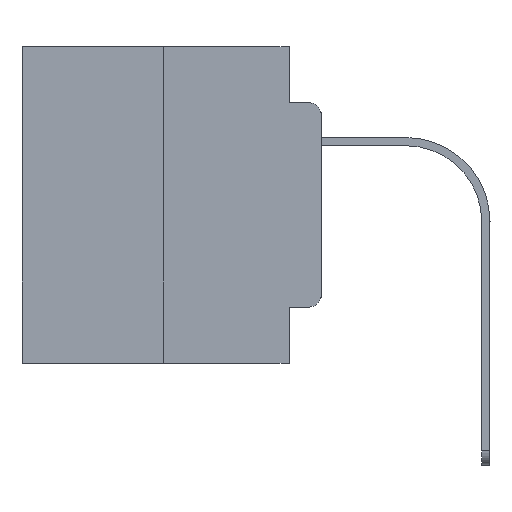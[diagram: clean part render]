
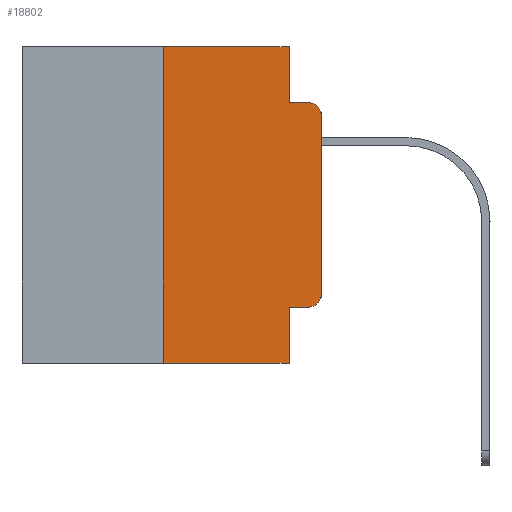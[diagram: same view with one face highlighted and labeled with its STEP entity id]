
A CAD part, left-side view. The second image highlights one B-rep face of the part: STEP entity #18802.
In plain terms, the highlighted planar face has unit normal (-1, 0, 0).
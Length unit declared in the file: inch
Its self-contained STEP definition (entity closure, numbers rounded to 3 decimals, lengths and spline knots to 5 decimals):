
#91 = AXIS2_PLACEMENT_3D ( 'NONE', #1571, #3238, #13882 ) ;
#158 = LINE ( 'NONE', #8084, #26917 ) ;
#404 = EDGE_CURVE ( 'NONE', #3718, #3940, #21538, .T. ) ;
#651 = CARTESIAN_POINT ( 'NONE',  ( 0., 0.051, -0.0885 ) ) ;
#1571 = CARTESIAN_POINT ( 'NONE',  ( 0., 0.02, -0.1085 ) ) ;
#2907 = CARTESIAN_POINT ( 'NONE',  ( 0., 0.051, 0. ) ) ;
#2915 = VECTOR ( 'NONE', #13723, 39.37008 ) ;
#3058 = DIRECTION ( 'NONE',  ( 0., 0., -1. ) ) ;
#3238 = DIRECTION ( 'NONE',  ( -1., 0., 0. ) ) ;
#3377 = LINE ( 'NONE', #20069, #20087 ) ;
#3543 = VECTOR ( 'NONE', #8685, 39.37008 ) ;
#3655 = DIRECTION ( 'NONE',  ( 0., 0., 1. ) ) ;
#3718 = VERTEX_POINT ( 'NONE', #19006 ) ;
#3940 = VERTEX_POINT ( 'NONE', #14063 ) ;
#4103 = EDGE_LOOP ( 'NONE', ( #11067, #22926, #19680, #26939, #23196, #11560, #5822, #4639, #4442, #11996 ) ) ;
#4203 = DIRECTION ( 'NONE',  ( 0., 0., 1. ) ) ;
#4442 = ORIENTED_EDGE ( 'NONE', *, *, #26563, .T. ) ;
#4639 = ORIENTED_EDGE ( 'NONE', *, *, #21658, .F. ) ;
#4985 = DIRECTION ( 'NONE',  ( -1., 0., 0. ) ) ;
#5822 = ORIENTED_EDGE ( 'NONE', *, *, #25167, .T. ) ;
#6753 = CARTESIAN_POINT ( 'NONE',  ( 0., 0.473, 0. ) ) ;
#7035 = EDGE_CURVE ( 'NONE', #16374, #21289, #8740, .T. ) ;
#7891 = VERTEX_POINT ( 'NONE', #25491 ) ;
#7911 = PLANE ( 'NONE',  #25468 ) ;
#8084 = CARTESIAN_POINT ( 'NONE',  ( 0., 0.051, 0. ) ) ;
#8685 = DIRECTION ( 'NONE',  ( 0., -1., 0. ) ) ;
#8740 = LINE ( 'NONE', #651, #23123 ) ;
#9224 = CARTESIAN_POINT ( 'NONE',  ( 0., 0.25, -0.5 ) ) ;
#9489 = EDGE_CURVE ( 'NONE', #19883, #19780, #26986, .T. ) ;
#9616 = CARTESIAN_POINT ( 'NONE',  ( 0., 0.02, -0.4115 ) ) ;
#10016 = VECTOR ( 'NONE', #23306, 39.37008 ) ;
#10236 = DIRECTION ( 'NONE',  ( 0., 0., -1. ) ) ;
#10416 = AXIS2_PLACEMENT_3D ( 'NONE', #21252, #4985, #23995 ) ;
#10860 = CARTESIAN_POINT ( 'NONE',  ( 0., 0.473, -0.5 ) ) ;
#11067 = ORIENTED_EDGE ( 'NONE', *, *, #15582, .T. ) ;
#11109 = CARTESIAN_POINT ( 'NONE',  ( 0., 0., -0.3915 ) ) ;
#11114 = CARTESIAN_POINT ( 'NONE',  ( 0., 0.02, -0.0885 ) ) ;
#11170 = EDGE_CURVE ( 'NONE', #3940, #16374, #25758, .T. ) ;
#11560 = ORIENTED_EDGE ( 'NONE', *, *, #18896, .F. ) ;
#11996 = ORIENTED_EDGE ( 'NONE', *, *, #9489, .T. ) ;
#12743 = VERTEX_POINT ( 'NONE', #9224 ) ;
#13083 = VECTOR ( 'NONE', #3058, 39.37008 ) ;
#13723 = DIRECTION ( 'NONE',  ( 0., -1., 0. ) ) ;
#13766 = CARTESIAN_POINT ( 'NONE',  ( 0., 0.051, -0.5 ) ) ;
#13882 = DIRECTION ( 'NONE',  ( 0., 0., -1. ) ) ;
#14063 = CARTESIAN_POINT ( 'NONE',  ( 0., 0.051, 0. ) ) ;
#14596 = LINE ( 'NONE', #22945, #16288 ) ;
#15122 = LINE ( 'NONE', #17966, #2915 ) ;
#15337 = CARTESIAN_POINT ( 'NONE',  ( 0., 0., -0.1085 ) ) ;
#15582 = EDGE_CURVE ( 'NONE', #19780, #20850, #3377, .T. ) ;
#16288 = VECTOR ( 'NONE', #4203, 39.37008 ) ;
#16374 = VERTEX_POINT ( 'NONE', #23965 ) ;
#16509 = DIRECTION ( 'NONE',  ( 1., 0., 0. ) ) ;
#17778 = EDGE_CURVE ( 'NONE', #20850, #21289, #19753, .T. ) ;
#17966 = CARTESIAN_POINT ( 'NONE',  ( 0., 0.051, -0.4115 ) ) ;
#18699 = CARTESIAN_POINT ( 'NONE',  ( 0., 0.473, 0. ) ) ;
#18802 = ADVANCED_FACE ( 'NONE', ( #26644 ), #7911, .F. ) ;
#18896 = EDGE_CURVE ( 'NONE', #12743, #3718, #14596, .T. ) ;
#19006 = CARTESIAN_POINT ( 'NONE',  ( 0., 0.25, 0. ) ) ;
#19680 = ORIENTED_EDGE ( 'NONE', *, *, #7035, .F. ) ;
#19753 = CIRCLE ( 'NONE', #91, 0.02 ) ;
#19780 = VERTEX_POINT ( 'NONE', #11109 ) ;
#19883 = VERTEX_POINT ( 'NONE', #9616 ) ;
#20069 = CARTESIAN_POINT ( 'NONE',  ( 0., 0., 0. ) ) ;
#20087 = VECTOR ( 'NONE', #3655, 39.37008 ) ;
#20850 = VERTEX_POINT ( 'NONE', #15337 ) ;
#21252 = CARTESIAN_POINT ( 'NONE',  ( 0., 0.02, -0.3915 ) ) ;
#21289 = VERTEX_POINT ( 'NONE', #11114 ) ;
#21538 = LINE ( 'NONE', #6753, #3543 ) ;
#21658 = EDGE_CURVE ( 'NONE', #7891, #23661, #158, .T. ) ;
#22926 = ORIENTED_EDGE ( 'NONE', *, *, #17778, .T. ) ;
#22945 = CARTESIAN_POINT ( 'NONE',  ( 0., 0.25, 0. ) ) ;
#22992 = DIRECTION ( 'NONE',  ( 0., 0., -1. ) ) ;
#23123 = VECTOR ( 'NONE', #23628, 39.37008 ) ;
#23196 = ORIENTED_EDGE ( 'NONE', *, *, #404, .F. ) ;
#23306 = DIRECTION ( 'NONE',  ( 0., -1., 0. ) ) ;
#23628 = DIRECTION ( 'NONE',  ( 0., -1., 0. ) ) ;
#23661 = VERTEX_POINT ( 'NONE', #13766 ) ;
#23965 = CARTESIAN_POINT ( 'NONE',  ( 0., 0.051, -0.0885 ) ) ;
#23995 = DIRECTION ( 'NONE',  ( 0., 0., -1. ) ) ;
#25167 = EDGE_CURVE ( 'NONE', #12743, #23661, #25374, .T. ) ;
#25374 = LINE ( 'NONE', #10860, #10016 ) ;
#25468 = AXIS2_PLACEMENT_3D ( 'NONE', #18699, #16509, #10236 ) ;
#25491 = CARTESIAN_POINT ( 'NONE',  ( 0., 0.051, -0.4115 ) ) ;
#25758 = LINE ( 'NONE', #2907, #13083 ) ;
#26563 = EDGE_CURVE ( 'NONE', #7891, #19883, #15122, .T. ) ;
#26644 = FACE_OUTER_BOUND ( 'NONE', #4103, .T. ) ;
#26917 = VECTOR ( 'NONE', #22992, 39.37008 ) ;
#26939 = ORIENTED_EDGE ( 'NONE', *, *, #11170, .F. ) ;
#26986 = CIRCLE ( 'NONE', #10416, 0.02 ) ;
